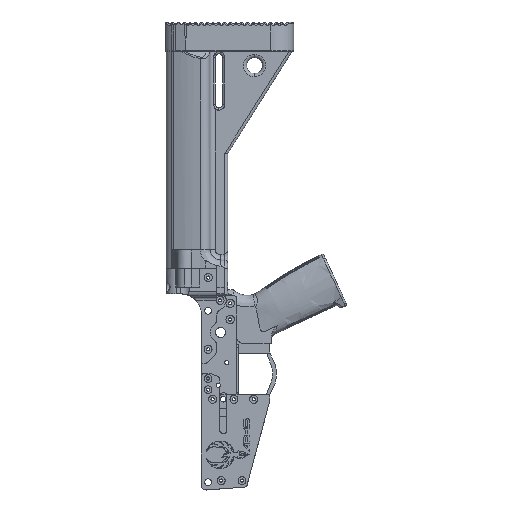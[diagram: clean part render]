
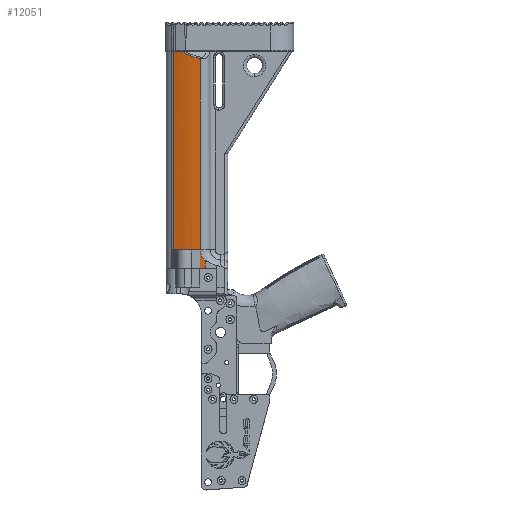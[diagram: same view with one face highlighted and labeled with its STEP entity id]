
A CAD part, left-side view. The second image highlights one B-rep face of the part: STEP entity #12051.
In plain terms, the highlighted cylindrical face has radius 104.245 mm (diameter 208.491 mm), a partial arc.
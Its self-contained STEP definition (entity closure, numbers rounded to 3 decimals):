
#186 = VERTEX_POINT ( 'NONE', #40039 ) ;
#1108 = VECTOR ( 'NONE', #74572, 1000. ) ;
#2482 = CARTESIAN_POINT ( 'NONE',  ( -20.34, 3.516, 216.269 ) ) ;
#5085 = CARTESIAN_POINT ( 'NONE',  ( -24.758, -17.002, 21.259 ) ) ;
#8330 = DIRECTION ( 'NONE',  ( 0., 0., 1. ) ) ;
#12051 = ADVANCED_FACE ( 'NONE', ( #144017 ), #62283, .T. ) ;
#13120 = CARTESIAN_POINT ( 'NONE',  ( -19.604, 5.788, 216.269 ) ) ;
#13181 = EDGE_CURVE ( 'NONE', #83943, #104711, #142564, .T. ) ;
#14771 = LINE ( 'NONE', #146871, #1108 ) ;
#15124 = VERTEX_POINT ( 'NONE', #80664 ) ;
#16870 = CARTESIAN_POINT ( 'NONE',  ( -24.922, -18.574, 18.828 ) ) ;
#17200 = EDGE_CURVE ( 'NONE', #108059, #186, #119159, .T. ) ;
#21292 = ORIENTED_EDGE ( 'NONE', *, *, #22956, .T. ) ;
#22956 = EDGE_CURVE ( 'NONE', #104711, #33086, #40422, .T. ) ;
#24468 = DIRECTION ( 'NONE',  ( 0., 0., -1. ) ) ;
#25830 = CARTESIAN_POINT ( 'NONE',  ( -23.293, -6.025, 28.806 ) ) ;
#26566 = VERTEX_POINT ( 'NONE', #33097 ) ;
#29442 = CARTESIAN_POINT ( 'NONE',  ( -24.993, -19.348, 17.887 ) ) ;
#30216 = CARTESIAN_POINT ( 'NONE',  ( -24.681, -16.328, 22.67 ) ) ;
#33070 = AXIS2_PLACEMENT_3D ( 'NONE', #147112, #24468, #63811 ) ;
#33086 = VERTEX_POINT ( 'NONE', #51254 ) ;
#33097 = CARTESIAN_POINT ( 'NONE',  ( -24.448, -14.503, 11.224 ) ) ;
#37450 = CARTESIAN_POINT ( 'NONE',  ( -17.901, 10.252, 216.269 ) ) ;
#37852 = EDGE_CURVE ( 'NONE', #186, #15124, #14771, .T. ) ;
#38488 = CARTESIAN_POINT ( 'NONE',  ( -25., -19.422, 17.806 ) ) ;
#40039 = CARTESIAN_POINT ( 'NONE',  ( -24.514, -14.997, 29.224 ) ) ;
#40422 = LINE ( 'NONE', #89182, #61624 ) ;
#40550 = CARTESIAN_POINT ( 'NONE',  ( -18.791, 8.035, 216.269 ) ) ;
#42011 = CARTESIAN_POINT ( 'NONE',  ( -24.845, -17.807, 19.901 ) ) ;
#42785 = CARTESIAN_POINT ( 'NONE',  ( -24.787, -17.256, 20.801 ) ) ;
#43564 = CARTESIAN_POINT ( 'NONE',  ( -24.983, -19.227, 18.024 ) ) ;
#45908 = CIRCLE ( 'NONE', #68601, 104.245 ) ;
#46661 = EDGE_CURVE ( 'NONE', #15124, #83943, #141775, .T. ) ;
#48674 = CARTESIAN_POINT ( 'NONE',  ( -17.901, 10.252, 28.806 ) ) ;
#50341 = CARTESIAN_POINT ( 'NONE',  ( -20.34, 3.516, 216.269 ) ) ;
#50965 = EDGE_CURVE ( 'NONE', #112823, #108059, #62035, .T. ) ;
#51254 = CARTESIAN_POINT ( 'NONE',  ( -17.901, 10.252, 28.806 ) ) ;
#53084 = CARTESIAN_POINT ( 'NONE',  ( -24.612, -15.759, 24.133 ) ) ;
#54624 = CARTESIAN_POINT ( 'NONE',  ( -24.527, -15.093, 27.162 ) ) ;
#56178 = CARTESIAN_POINT ( 'NONE',  ( -24.954, -18.917, 18.398 ) ) ;
#61624 = VECTOR ( 'NONE', #148953, 1000. ) ;
#62035 = B_SPLINE_CURVE_WITH_KNOTS ( 'NONE', 3,
 ( #132109, #98316, #146216, #38488 ),
 .UNSPECIFIED., .F., .F.,
 ( 4, 4 ),
 ( 0., 1. ),
 .UNSPECIFIED. ) ;
#62283 = CYLINDRICAL_SURFACE ( 'NONE', #33070, 104.245 ) ;
#62297 = CARTESIAN_POINT ( 'NONE',  ( -23.695, -8.76, 210.62 ) ) ;
#63811 = DIRECTION ( 'NONE',  ( -1., 0., 0. ) ) ;
#66304 = LINE ( 'NONE', #78852, #120044 ) ;
#66436 = CARTESIAN_POINT ( 'NONE',  ( -24.576, -15.475, 25.127 ) ) ;
#68601 = AXIS2_PLACEMENT_3D ( 'NONE', #105878, #8330, #117675 ) ;
#74572 = DIRECTION ( 'NONE',  ( 0., 0., 1. ) ) ;
#76461 = ORIENTED_EDGE ( 'NONE', *, *, #37852, .T. ) ;
#76668 = CARTESIAN_POINT ( 'NONE',  ( -24.961, -18.989, 18.309 ) ) ;
#77438 = CARTESIAN_POINT ( 'NONE',  ( -24.955, -18.929, 18.383 ) ) ;
#78852 = CARTESIAN_POINT ( 'NONE',  ( -24.448, -14.503, 10.825 ) ) ;
#80664 = CARTESIAN_POINT ( 'NONE',  ( -24.514, -14.997, 209.24 ) ) ;
#83612 = VERTEX_POINT ( 'NONE', #108946 ) ;
#83943 = VERTEX_POINT ( 'NONE', #50341 ) ;
#89182 = CARTESIAN_POINT ( 'NONE',  ( -17.901, 10.252, 10.825 ) ) ;
#90595 = ORIENTED_EDGE ( 'NONE', *, *, #50965, .T. ) ;
#90613 = ORIENTED_EDGE ( 'NONE', *, *, #111914, .T. ) ;
#91557 = CARTESIAN_POINT ( 'NONE',  ( -24.957, -18.947, 18.36 ) ) ;
#94920 = ORIENTED_EDGE ( 'NONE', *, *, #103961, .T. ) ;
#98316 = CARTESIAN_POINT ( 'NONE',  ( -25., -19.422, 13.418 ) ) ;
#103961 = EDGE_CURVE ( 'NONE', #83612, #26566, #66304, .T. ) ;
#104711 = VERTEX_POINT ( 'NONE', #105254 ) ;
#105254 = CARTESIAN_POINT ( 'NONE',  ( -17.901, 10.252, 216.269 ) ) ;
#105739 = CARTESIAN_POINT ( 'NONE',  ( -24.514, -14.997, 29.224 ) ) ;
#105878 = CARTESIAN_POINT ( 'NONE',  ( 78.842, -28.578, 11.224 ) ) ;
#108059 = VERTEX_POINT ( 'NONE', #111210 ) ;
#108323 = CARTESIAN_POINT ( 'NONE',  ( -20.34, 3.516, 216.269 ) ) ;
#108472 = CARTESIAN_POINT ( 'NONE',  ( -21.089, 2.311, 28.806 ) ) ;
#108946 = CARTESIAN_POINT ( 'NONE',  ( -24.448, -14.503, 28.806 ) ) ;
#111210 = CARTESIAN_POINT ( 'NONE',  ( -25., -19.422, 17.806 ) ) ;
#111351 = ORIENTED_EDGE ( 'NONE', *, *, #46661, .T. ) ;
#111914 = EDGE_CURVE ( 'NONE', #26566, #112823, #45908, .T. ) ;
#112823 = VERTEX_POINT ( 'NONE', #134130 ) ;
#112876 = CARTESIAN_POINT ( 'NONE',  ( -24.876, -18.102, 19.465 ) ) ;
#117675 = DIRECTION ( 'NONE',  ( -1., 0., 0. ) ) ;
#119159 = B_SPLINE_CURVE_WITH_KNOTS ( 'NONE', 3,
 ( #151320, #29442, #43564, #149768, #76668, #91557, #77438, #56178, #150544, #124646, #16870, #112876, #42011, #42785, #5085, #137957, #30216, #53084, #66436, #54624, #143388, #105739 ),
 .UNSPECIFIED., .F., .F.,
 ( 4, 1, 1, 1, 1, 2, 2, 2, 2, 2, 2, 2, 4 ),
 ( 0., 0.031, 0.047, 0.055, 0.059, 0.061, 0.062, 0.125, 0.25, 0.375, 0.5, 0.75, 1. ),
 .UNSPECIFIED. ) ;
#120044 = VECTOR ( 'NONE', #139368, 1000. ) ;
#124646 = CARTESIAN_POINT ( 'NONE',  ( -24.937, -18.737, 18.618 ) ) ;
#126734 = EDGE_LOOP ( 'NONE', ( #94920, #90613, #90595, #147652, #76461, #111351, #131786, #21292, #135270 ) ) ;
#128600 = B_SPLINE_CURVE_WITH_KNOTS ( 'NONE', 3,
 ( #48674, #108472, #25830, #142251 ),
 .UNSPECIFIED., .F., .F.,
 ( 4, 4 ),
 ( 0., 1. ),
 .UNSPECIFIED. ) ;
#131786 = ORIENTED_EDGE ( 'NONE', *, *, #13181, .T. ) ;
#132109 = CARTESIAN_POINT ( 'NONE',  ( -25., -19.422, 11.224 ) ) ;
#133357 = EDGE_CURVE ( 'NONE', #33086, #83612, #128600, .T. ) ;
#134130 = CARTESIAN_POINT ( 'NONE',  ( -25., -19.422, 11.224 ) ) ;
#135270 = ORIENTED_EDGE ( 'NONE', *, *, #133357, .T. ) ;
#136118 = CARTESIAN_POINT ( 'NONE',  ( -22.303, -2.553, 212.964 ) ) ;
#137957 = CARTESIAN_POINT ( 'NONE',  ( -24.705, -16.538, 22.195 ) ) ;
#139368 = DIRECTION ( 'NONE',  ( 0., 0., -1. ) ) ;
#141775 = B_SPLINE_CURVE_WITH_KNOTS ( 'NONE', 3,
 ( #146360, #62297, #136118, #2482 ),
 .UNSPECIFIED., .F., .F.,
 ( 4, 4 ),
 ( 0., 1. ),
 .UNSPECIFIED. ) ;
#142251 = CARTESIAN_POINT ( 'NONE',  ( -24.448, -14.503, 28.806 ) ) ;
#142564 = B_SPLINE_CURVE_WITH_KNOTS ( 'NONE', 3,
 ( #108323, #13120, #40550, #37450 ),
 .UNSPECIFIED., .F., .F.,
 ( 4, 4 ),
 ( 0., 1. ),
 .UNSPECIFIED. ) ;
#143388 = CARTESIAN_POINT ( 'NONE',  ( -24.514, -14.997, 28.188 ) ) ;
#144017 = FACE_OUTER_BOUND ( 'NONE', #126734, .T. ) ;
#146216 = CARTESIAN_POINT ( 'NONE',  ( -25., -19.422, 15.612 ) ) ;
#146360 = CARTESIAN_POINT ( 'NONE',  ( -24.514, -14.997, 209.24 ) ) ;
#146871 = CARTESIAN_POINT ( 'NONE',  ( -24.514, -14.997, 10.825 ) ) ;
#147112 = CARTESIAN_POINT ( 'NONE',  ( 78.842, -28.578, 10.825 ) ) ;
#147652 = ORIENTED_EDGE ( 'NONE', *, *, #17200, .T. ) ;
#148953 = DIRECTION ( 'NONE',  ( 0., 0., -1. ) ) ;
#149768 = CARTESIAN_POINT ( 'NONE',  ( -24.968, -19.071, 18.21 ) ) ;
#150544 = CARTESIAN_POINT ( 'NONE',  ( -24.954, -18.91, 18.406 ) ) ;
#151320 = CARTESIAN_POINT ( 'NONE',  ( -25., -19.422, 17.806 ) ) ;
